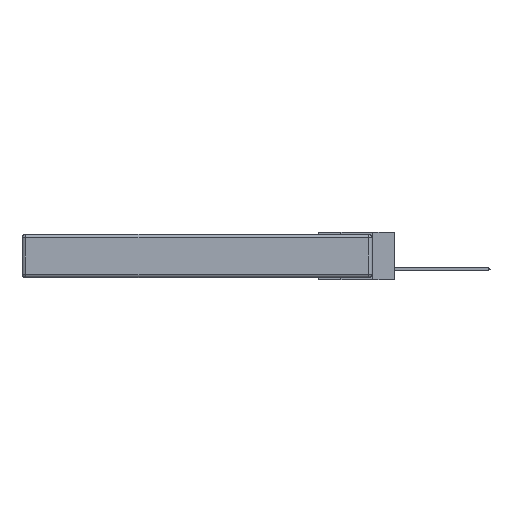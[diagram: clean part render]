
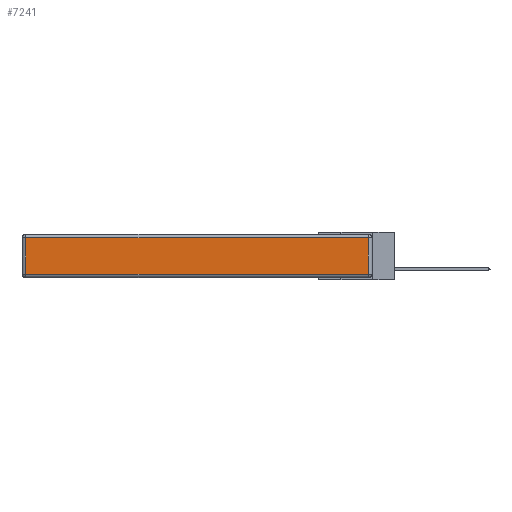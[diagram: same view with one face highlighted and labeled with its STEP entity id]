
A CAD part, left-side view. The second image highlights one B-rep face of the part: STEP entity #7241.
In plain terms, the highlighted planar face has unit normal (-1, 0, 0).
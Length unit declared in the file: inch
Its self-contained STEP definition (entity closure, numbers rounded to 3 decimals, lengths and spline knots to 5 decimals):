
#276 = LINE ( 'NONE', #15539, #14291 ) ;
#646 = LINE ( 'NONE', #5714, #1265 ) ;
#713 = CARTESIAN_POINT ( 'NONE',  ( 0., 0., -0.343 ) ) ;
#1265 = VECTOR ( 'NONE', #11698, 39.37008 ) ;
#2319 = FACE_OUTER_BOUND ( 'NONE', #11816, .T. ) ;
#2774 = EDGE_CURVE ( 'NONE', #22486, #14657, #22293, .T. ) ;
#2795 = DIRECTION ( 'NONE',  ( 0., 0., 1. ) ) ;
#4384 = DIRECTION ( 'NONE',  ( 0., 1., 0. ) ) ;
#4756 = LINE ( 'NONE', #15995, #13706 ) ;
#5714 = CARTESIAN_POINT ( 'NONE',  ( 0., 0.03, -0.343 ) ) ;
#5861 = ORIENTED_EDGE ( 'NONE', *, *, #2774, .T. ) ;
#7241 = ADVANCED_FACE ( 'NONE', ( #2319 ), #10538, .T. ) ;
#7276 = CARTESIAN_POINT ( 'NONE',  ( 0., 2.72, -0.343 ) ) ;
#7610 = DIRECTION ( 'NONE',  ( 0., 0., -1. ) ) ;
#9475 = VECTOR ( 'NONE', #7610, 39.37008 ) ;
#10538 = PLANE ( 'NONE',  #22873 ) ;
#11698 = DIRECTION ( 'NONE',  ( 0., 0., 1. ) ) ;
#11816 = EDGE_LOOP ( 'NONE', ( #22211, #22924, #22093, #5861 ) ) ;
#12899 = VERTEX_POINT ( 'NONE', #24640 ) ;
#13706 = VECTOR ( 'NONE', #23834, 39.37008 ) ;
#14291 = VECTOR ( 'NONE', #4384, 39.37008 ) ;
#14657 = VERTEX_POINT ( 'NONE', #16977 ) ;
#15057 = EDGE_CURVE ( 'NONE', #16874, #22486, #276, .T. ) ;
#15539 = CARTESIAN_POINT ( 'NONE',  ( 0., 2.75, -0.03 ) ) ;
#15995 = CARTESIAN_POINT ( 'NONE',  ( 0., 0., -0.313 ) ) ;
#16874 = VERTEX_POINT ( 'NONE', #23239 ) ;
#16977 = CARTESIAN_POINT ( 'NONE',  ( 0., 2.72, -0.313 ) ) ;
#18038 = DIRECTION ( 'NONE',  ( -1., 0., 0. ) ) ;
#22093 = ORIENTED_EDGE ( 'NONE', *, *, #15057, .T. ) ;
#22211 = ORIENTED_EDGE ( 'NONE', *, *, #24018, .T. ) ;
#22293 = LINE ( 'NONE', #7276, #9475 ) ;
#22486 = VERTEX_POINT ( 'NONE', #23068 ) ;
#22766 = EDGE_CURVE ( 'NONE', #12899, #16874, #646, .T. ) ;
#22873 = AXIS2_PLACEMENT_3D ( 'NONE', #713, #18038, #2795 ) ;
#22924 = ORIENTED_EDGE ( 'NONE', *, *, #22766, .T. ) ;
#23068 = CARTESIAN_POINT ( 'NONE',  ( 0., 2.72, -0.03 ) ) ;
#23239 = CARTESIAN_POINT ( 'NONE',  ( 0., 0.03, -0.03 ) ) ;
#23834 = DIRECTION ( 'NONE',  ( 0., -1., 0. ) ) ;
#24018 = EDGE_CURVE ( 'NONE', #14657, #12899, #4756, .T. ) ;
#24640 = CARTESIAN_POINT ( 'NONE',  ( 0., 0.03, -0.313 ) ) ;
